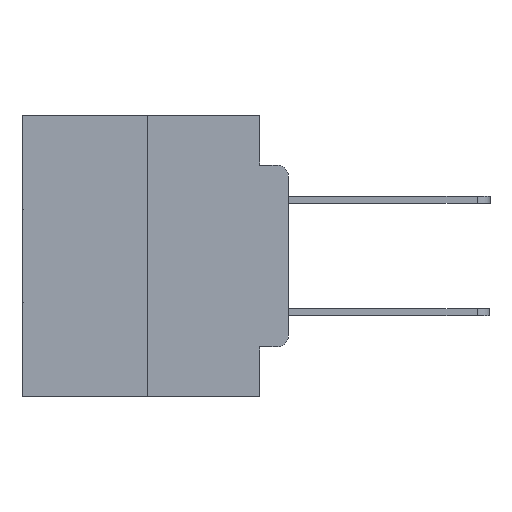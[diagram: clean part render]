
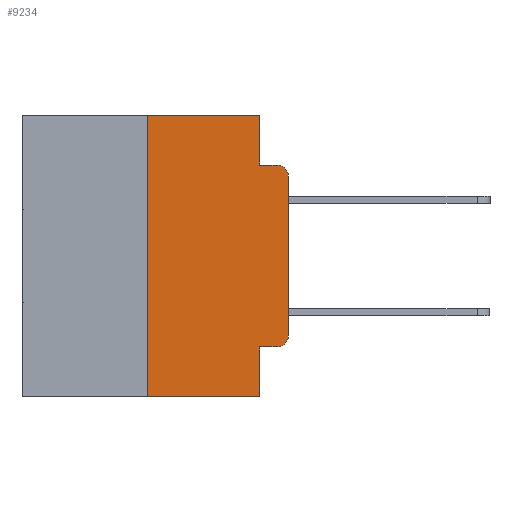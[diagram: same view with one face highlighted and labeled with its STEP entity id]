
A CAD part, left-side view. The second image highlights one B-rep face of the part: STEP entity #9234.
In plain terms, the highlighted planar face has unit normal (-1, 0, 0).
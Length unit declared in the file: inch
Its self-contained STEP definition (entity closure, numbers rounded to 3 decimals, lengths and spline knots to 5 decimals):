
#230 = VERTEX_POINT ( 'NONE', #11190 ) ;
#438 = LINE ( 'NONE', #25743, #5714 ) ;
#531 = VECTOR ( 'NONE', #17109, 39.37008 ) ;
#698 = EDGE_CURVE ( 'NONE', #6962, #230, #7749, .T. ) ;
#969 = ORIENTED_EDGE ( 'NONE', *, *, #698, .F. ) ;
#1101 = EDGE_CURVE ( 'NONE', #7809, #24603, #26229, .T. ) ;
#1367 = AXIS2_PLACEMENT_3D ( 'NONE', #2587, #17933, #4825 ) ;
#1581 = DIRECTION ( 'NONE',  ( 0., 0., -1. ) ) ;
#1970 = DIRECTION ( 'NONE',  ( 0., -1., 0. ) ) ;
#2258 = EDGE_CURVE ( 'NONE', #230, #23201, #15875, .T. ) ;
#2451 = CARTESIAN_POINT ( 'NONE',  ( 0., 0., -0.1085 ) ) ;
#2568 = VECTOR ( 'NONE', #5335, 39.37008 ) ;
#2587 = CARTESIAN_POINT ( 'NONE',  ( 0., 0.473, 0. ) ) ;
#3055 = CARTESIAN_POINT ( 'NONE',  ( 0., 0.25, 0. ) ) ;
#3104 = CARTESIAN_POINT ( 'NONE',  ( 0., 0.051, 0. ) ) ;
#3146 = VERTEX_POINT ( 'NONE', #3055 ) ;
#3814 = ORIENTED_EDGE ( 'NONE', *, *, #22850, .F. ) ;
#4825 = DIRECTION ( 'NONE',  ( 0., 0., -1. ) ) ;
#5192 = VERTEX_POINT ( 'NONE', #20699 ) ;
#5207 = EDGE_CURVE ( 'NONE', #9722, #23201, #22137, .T. ) ;
#5335 = DIRECTION ( 'NONE',  ( 0., 0., -1. ) ) ;
#5714 = VECTOR ( 'NONE', #1970, 39.37008 ) ;
#5815 = CARTESIAN_POINT ( 'NONE',  ( 0., 0.051, 0. ) ) ;
#5882 = ORIENTED_EDGE ( 'NONE', *, *, #23188, .F. ) ;
#6099 = CIRCLE ( 'NONE', #20249, 0.02 ) ;
#6581 = DIRECTION ( 'NONE',  ( 0., 0., 1. ) ) ;
#6631 = CARTESIAN_POINT ( 'NONE',  ( 0., 0.25, -0.5 ) ) ;
#6704 = EDGE_CURVE ( 'NONE', #12840, #9722, #23732, .T. ) ;
#6962 = VERTEX_POINT ( 'NONE', #5815 ) ;
#7059 = FACE_OUTER_BOUND ( 'NONE', #17254, .T. ) ;
#7187 = DIRECTION ( 'NONE',  ( -1., 0., 0. ) ) ;
#7749 = LINE ( 'NONE', #23722, #18656 ) ;
#7809 = VERTEX_POINT ( 'NONE', #6631 ) ;
#7861 = CARTESIAN_POINT ( 'NONE',  ( 0., 0., -0.3915 ) ) ;
#8489 = CARTESIAN_POINT ( 'NONE',  ( 0., 0.051, -0.5 ) ) ;
#8972 = DIRECTION ( 'NONE',  ( 0., -1., 0. ) ) ;
#9234 = ADVANCED_FACE ( 'NONE', ( #7059 ), #15751, .F. ) ;
#9722 = VERTEX_POINT ( 'NONE', #2451 ) ;
#9771 = CARTESIAN_POINT ( 'NONE',  ( 0., 0.02, -0.0885 ) ) ;
#11190 = CARTESIAN_POINT ( 'NONE',  ( 0., 0.051, -0.0885 ) ) ;
#12239 = CARTESIAN_POINT ( 'NONE',  ( 0., 0.02, -0.1085 ) ) ;
#12840 = VERTEX_POINT ( 'NONE', #7861 ) ;
#13300 = CARTESIAN_POINT ( 'NONE',  ( 0., 0.473, -0.5 ) ) ;
#13951 = VECTOR ( 'NONE', #21727, 39.37008 ) ;
#14421 = DIRECTION ( 'NONE',  ( 0., 0., -1. ) ) ;
#14934 = VECTOR ( 'NONE', #8972, 39.37008 ) ;
#15751 = PLANE ( 'NONE',  #1367 ) ;
#15875 = LINE ( 'NONE', #19564, #22180 ) ;
#17109 = DIRECTION ( 'NONE',  ( 0., 0., 1. ) ) ;
#17254 = EDGE_LOOP ( 'NONE', ( #22115, #27780, #23475, #969, #3814, #26767, #22460, #5882, #18865, #24476 ) ) ;
#17489 = CARTESIAN_POINT ( 'NONE',  ( 0., 0.25, 0. ) ) ;
#17933 = DIRECTION ( 'NONE',  ( 1., 0., 0. ) ) ;
#18176 = VERTEX_POINT ( 'NONE', #27430 ) ;
#18656 = VECTOR ( 'NONE', #1581, 39.37008 ) ;
#18865 = ORIENTED_EDGE ( 'NONE', *, *, #21760, .T. ) ;
#19564 = CARTESIAN_POINT ( 'NONE',  ( 0., 0.051, -0.0885 ) ) ;
#19876 = LINE ( 'NONE', #17489, #24828 ) ;
#20199 = CARTESIAN_POINT ( 'NONE',  ( 0., 0.02, -0.3915 ) ) ;
#20249 = AXIS2_PLACEMENT_3D ( 'NONE', #20199, #7187, #22309 ) ;
#20340 = EDGE_CURVE ( 'NONE', #18176, #12840, #6099, .T. ) ;
#20651 = LINE ( 'NONE', #3104, #2568 ) ;
#20699 = CARTESIAN_POINT ( 'NONE',  ( 0., 0.051, -0.4115 ) ) ;
#21727 = DIRECTION ( 'NONE',  ( 0., -1., 0. ) ) ;
#21760 = EDGE_CURVE ( 'NONE', #5192, #18176, #25286, .T. ) ;
#22097 = AXIS2_PLACEMENT_3D ( 'NONE', #12239, #27161, #14421 ) ;
#22115 = ORIENTED_EDGE ( 'NONE', *, *, #6704, .T. ) ;
#22137 = CIRCLE ( 'NONE', #22097, 0.02 ) ;
#22180 = VECTOR ( 'NONE', #27962, 39.37008 ) ;
#22309 = DIRECTION ( 'NONE',  ( 0., 0., -1. ) ) ;
#22460 = ORIENTED_EDGE ( 'NONE', *, *, #1101, .T. ) ;
#22850 = EDGE_CURVE ( 'NONE', #3146, #6962, #438, .T. ) ;
#23188 = EDGE_CURVE ( 'NONE', #5192, #24603, #20651, .T. ) ;
#23201 = VERTEX_POINT ( 'NONE', #9771 ) ;
#23475 = ORIENTED_EDGE ( 'NONE', *, *, #2258, .F. ) ;
#23722 = CARTESIAN_POINT ( 'NONE',  ( 0., 0.051, 0. ) ) ;
#23732 = LINE ( 'NONE', #27649, #531 ) ;
#24476 = ORIENTED_EDGE ( 'NONE', *, *, #20340, .T. ) ;
#24603 = VERTEX_POINT ( 'NONE', #8489 ) ;
#24828 = VECTOR ( 'NONE', #6581, 39.37008 ) ;
#25286 = LINE ( 'NONE', #28025, #13951 ) ;
#25743 = CARTESIAN_POINT ( 'NONE',  ( 0., 0.473, 0. ) ) ;
#26002 = EDGE_CURVE ( 'NONE', #7809, #3146, #19876, .T. ) ;
#26229 = LINE ( 'NONE', #13300, #14934 ) ;
#26767 = ORIENTED_EDGE ( 'NONE', *, *, #26002, .F. ) ;
#27161 = DIRECTION ( 'NONE',  ( -1., 0., 0. ) ) ;
#27430 = CARTESIAN_POINT ( 'NONE',  ( 0., 0.02, -0.4115 ) ) ;
#27649 = CARTESIAN_POINT ( 'NONE',  ( 0., 0., 0. ) ) ;
#27780 = ORIENTED_EDGE ( 'NONE', *, *, #5207, .T. ) ;
#27962 = DIRECTION ( 'NONE',  ( 0., -1., 0. ) ) ;
#28025 = CARTESIAN_POINT ( 'NONE',  ( 0., 0.051, -0.4115 ) ) ;
